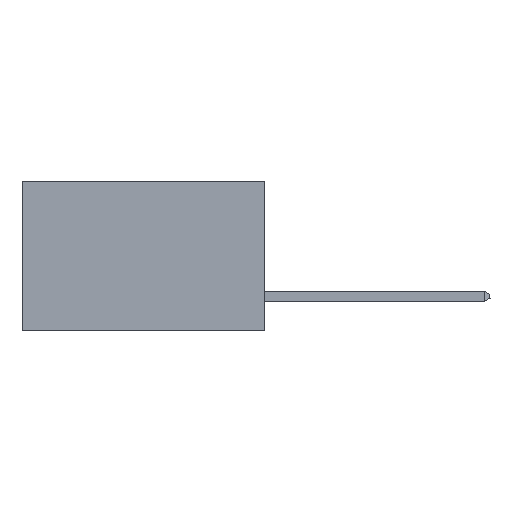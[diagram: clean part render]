
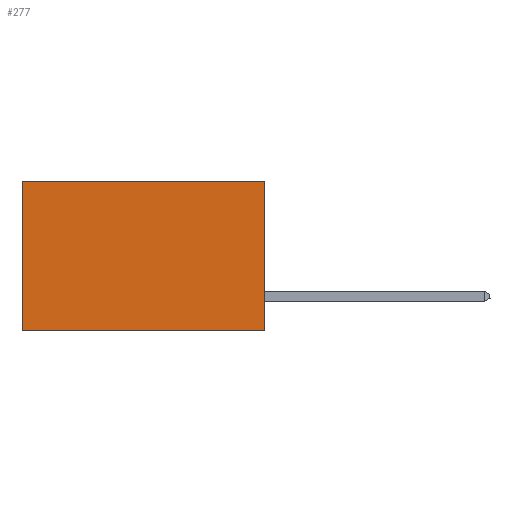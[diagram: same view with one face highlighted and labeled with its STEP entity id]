
A CAD part, left-side view. The second image highlights one B-rep face of the part: STEP entity #277.
In plain terms, the highlighted planar face has unit normal (-1, 0, 0).
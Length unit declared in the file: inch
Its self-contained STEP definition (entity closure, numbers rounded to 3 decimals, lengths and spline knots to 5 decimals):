
#41 = EDGE_CURVE ( 'NONE', #2744, #6742, #4614, .T. ) ;
#183 = ORIENTED_EDGE ( 'NONE', *, *, #7379, .F. ) ;
#277 = ADVANCED_FACE ( 'NONE', ( #360 ), #4868, .F. ) ;
#360 = FACE_OUTER_BOUND ( 'NONE', #6343, .T. ) ;
#860 = ORIENTED_EDGE ( 'NONE', *, *, #2289, .T. ) ;
#994 = CARTESIAN_POINT ( 'NONE',  ( 0.298, 0.6, 0. ) ) ;
#1227 = VERTEX_POINT ( 'NONE', #1936 ) ;
#1365 = DIRECTION ( 'NONE',  ( 0., 1., 0. ) ) ;
#1644 = DIRECTION ( 'NONE',  ( 0., 0., -1. ) ) ;
#1753 = DIRECTION ( 'NONE',  ( 0., 1., 0. ) ) ;
#1936 = CARTESIAN_POINT ( 'NONE',  ( 0.298, 0., 0. ) ) ;
#2289 = EDGE_CURVE ( 'NONE', #1227, #5123, #6142, .T. ) ;
#2443 = CARTESIAN_POINT ( 'NONE',  ( 0.298, 0., 0. ) ) ;
#2744 = VERTEX_POINT ( 'NONE', #8888 ) ;
#2940 = VECTOR ( 'NONE', #1753, 39.37008 ) ;
#3205 = CARTESIAN_POINT ( 'NONE',  ( 0.298, 0., -0.37 ) ) ;
#3273 = DIRECTION ( 'NONE',  ( 1., 0., 0. ) ) ;
#3304 = CARTESIAN_POINT ( 'NONE',  ( 0.298, 0.6, -0.37 ) ) ;
#3321 = LINE ( 'NONE', #994, #4983 ) ;
#3407 = LINE ( 'NONE', #2443, #5937 ) ;
#3431 = ORIENTED_EDGE ( 'NONE', *, *, #6082, .T. ) ;
#4614 = LINE ( 'NONE', #3205, #2940 ) ;
#4746 = CARTESIAN_POINT ( 'NONE',  ( 0.298, 0., 0. ) ) ;
#4823 = AXIS2_PLACEMENT_3D ( 'NONE', #4746, #3273, #1644 ) ;
#4868 = PLANE ( 'NONE',  #4823 ) ;
#4901 = DIRECTION ( 'NONE',  ( 0., 0., -1. ) ) ;
#4983 = VECTOR ( 'NONE', #4901, 39.37008 ) ;
#5123 = VERTEX_POINT ( 'NONE', #6724 ) ;
#5937 = VECTOR ( 'NONE', #9425, 39.37008 ) ;
#6082 = EDGE_CURVE ( 'NONE', #5123, #6742, #3321, .T. ) ;
#6142 = LINE ( 'NONE', #9979, #7233 ) ;
#6343 = EDGE_LOOP ( 'NONE', ( #3431, #7226, #183, #860 ) ) ;
#6724 = CARTESIAN_POINT ( 'NONE',  ( 0.298, 0.6, 0. ) ) ;
#6742 = VERTEX_POINT ( 'NONE', #3304 ) ;
#7226 = ORIENTED_EDGE ( 'NONE', *, *, #41, .F. ) ;
#7233 = VECTOR ( 'NONE', #1365, 39.37008 ) ;
#7379 = EDGE_CURVE ( 'NONE', #1227, #2744, #3407, .T. ) ;
#8888 = CARTESIAN_POINT ( 'NONE',  ( 0.298, 0., -0.37 ) ) ;
#9425 = DIRECTION ( 'NONE',  ( 0., 0., -1. ) ) ;
#9979 = CARTESIAN_POINT ( 'NONE',  ( 0.298, 0., 0. ) ) ;
